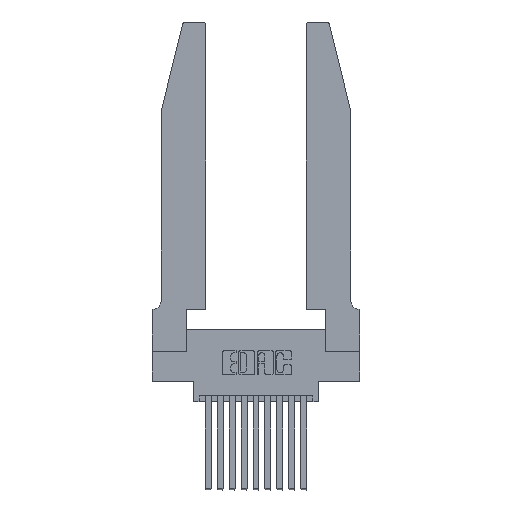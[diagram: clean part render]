
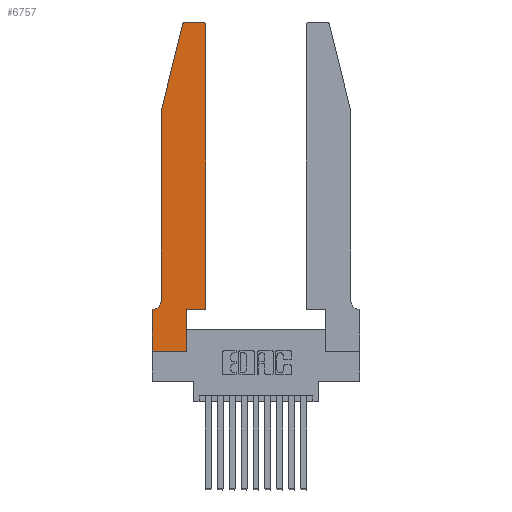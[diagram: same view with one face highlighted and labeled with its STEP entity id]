
A CAD part, top view. The second image highlights one B-rep face of the part: STEP entity #6757.
In plain terms, the highlighted planar face has unit normal (0, 0, 1).
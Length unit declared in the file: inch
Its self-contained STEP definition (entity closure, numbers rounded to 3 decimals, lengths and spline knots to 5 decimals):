
#360 = EDGE_CURVE ( 'NONE', #2141, #6995, #12577, .T. ) ;
#584 = EDGE_CURVE ( 'NONE', #11350, #10825, #13136, .T. ) ;
#772 = VERTEX_POINT ( 'NONE', #2918 ) ;
#892 = VECTOR ( 'NONE', #13113, 39.37008 ) ;
#911 = EDGE_CURVE ( 'NONE', #772, #13180, #12179, .T. ) ;
#1181 = CARTESIAN_POINT ( 'NONE',  ( 0.4205, 2.72, 0.37 ) ) ;
#1663 = DIRECTION ( 'NONE',  ( 0., 1., 0. ) ) ;
#1687 = ORIENTED_EDGE ( 'NONE', *, *, #360, .T. ) ;
#1718 = LINE ( 'NONE', #3929, #2620 ) ;
#1824 = VERTEX_POINT ( 'NONE', #14068 ) ;
#1934 = LINE ( 'NONE', #10554, #11210 ) ;
#2077 = EDGE_CURVE ( 'NONE', #1824, #2141, #7849, .T. ) ;
#2141 = VERTEX_POINT ( 'NONE', #2347 ) ;
#2347 = CARTESIAN_POINT ( 'NONE',  ( 0.4205, 2.75, 0.37 ) ) ;
#2473 = VERTEX_POINT ( 'NONE', #11221 ) ;
#2587 = ORIENTED_EDGE ( 'NONE', *, *, #12162, .T. ) ;
#2606 = CARTESIAN_POINT ( 'NONE',  ( 0.4505, 0.35, 0.37 ) ) ;
#2620 = VECTOR ( 'NONE', #5188, 39.37008 ) ;
#2737 = CARTESIAN_POINT ( 'NONE',  ( 0.0055, 0.42, 0.37 ) ) ;
#2860 = VERTEX_POINT ( 'NONE', #4468 ) ;
#2918 = CARTESIAN_POINT ( 'NONE',  ( 0.0755, 2., 0.37 ) ) ;
#3276 = DIRECTION ( 'NONE',  ( 1., 0., 0. ) ) ;
#3290 = DIRECTION ( 'NONE',  ( 1., 0., 0. ) ) ;
#3381 = CARTESIAN_POINT ( 'NONE',  ( 0.284, 2.72, 0.37 ) ) ;
#3717 = VECTOR ( 'NONE', #14409, 39.37008 ) ;
#3866 = AXIS2_PLACEMENT_3D ( 'NONE', #2737, #11454, #4101 ) ;
#3867 = EDGE_CURVE ( 'NONE', #16018, #772, #12077, .T. ) ;
#3929 = CARTESIAN_POINT ( 'NONE',  ( 0., 0., 0.37 ) ) ;
#4035 = CARTESIAN_POINT ( 'NONE',  ( 0.0755, 2., 0.37 ) ) ;
#4101 = DIRECTION ( 'NONE',  ( -1., 0., 0. ) ) ;
#4468 = CARTESIAN_POINT ( 'NONE',  ( 0.2865, 0.35, 0.37 ) ) ;
#4697 = DIRECTION ( 'NONE',  ( 1., 0., 0. ) ) ;
#4889 = CARTESIAN_POINT ( 'NONE',  ( 0.0755, 0.42, 0.37 ) ) ;
#5188 = DIRECTION ( 'NONE',  ( 0., -1., 0. ) ) ;
#5638 = ORIENTED_EDGE ( 'NONE', *, *, #3867, .T. ) ;
#5704 = VECTOR ( 'NONE', #12519, 39.37008 ) ;
#5881 = EDGE_CURVE ( 'NONE', #2473, #1824, #9596, .T. ) ;
#6305 = VECTOR ( 'NONE', #10790, 39.37008 ) ;
#6439 = ORIENTED_EDGE ( 'NONE', *, *, #584, .T. ) ;
#6757 = ADVANCED_FACE ( 'NONE', ( #13494 ), #14294, .T. ) ;
#6842 = AXIS2_PLACEMENT_3D ( 'NONE', #1181, #14568, #3276 ) ;
#6995 = VERTEX_POINT ( 'NONE', #16111 ) ;
#7089 = LINE ( 'NONE', #13214, #3717 ) ;
#7103 = CARTESIAN_POINT ( 'NONE',  ( 0.0755, 0.35, 0.37 ) ) ;
#7469 = CIRCLE ( 'NONE', #10896, 0.03 ) ;
#7614 = EDGE_CURVE ( 'NONE', #10806, #11350, #1718, .T. ) ;
#7849 = CIRCLE ( 'NONE', #6842, 0.03 ) ;
#8258 = LINE ( 'NONE', #7103, #892 ) ;
#8334 = CARTESIAN_POINT ( 'NONE',  ( 0., 0.35, 0.37 ) ) ;
#8481 = CARTESIAN_POINT ( 'NONE',  ( 0.2605, 2.75, 0.37 ) ) ;
#8576 = ORIENTED_EDGE ( 'NONE', *, *, #13476, .T. ) ;
#8706 = CARTESIAN_POINT ( 'NONE',  ( 0., 0., 0.37 ) ) ;
#8830 = CARTESIAN_POINT ( 'NONE',  ( 0.25487, 2.72718, 0.37 ) ) ;
#8946 = ORIENTED_EDGE ( 'NONE', *, *, #911, .T. ) ;
#9067 = DIRECTION ( 'NONE',  ( -1., 0., 0. ) ) ;
#9222 = VECTOR ( 'NONE', #12546, 39.37008 ) ;
#9330 = ORIENTED_EDGE ( 'NONE', *, *, #12997, .T. ) ;
#9575 = CARTESIAN_POINT ( 'NONE',  ( 0.0755, 2., 0.37 ) ) ;
#9596 = LINE ( 'NONE', #2606, #9222 ) ;
#9603 = CIRCLE ( 'NONE', #3866, 0.07 ) ;
#9933 = CARTESIAN_POINT ( 'NONE',  ( 0., 0.35, 0.37 ) ) ;
#9950 = AXIS2_PLACEMENT_3D ( 'NONE', #8334, #10729, #3290 ) ;
#10070 = ORIENTED_EDGE ( 'NONE', *, *, #13066, .T. ) ;
#10554 = CARTESIAN_POINT ( 'NONE',  ( 0.2865, 0.35, 0.37 ) ) ;
#10729 = DIRECTION ( 'NONE',  ( 0., 0., 1. ) ) ;
#10790 = DIRECTION ( 'NONE',  ( 1., 0., 0. ) ) ;
#10806 = VERTEX_POINT ( 'NONE', #9933 ) ;
#10825 = VERTEX_POINT ( 'NONE', #15928 ) ;
#10896 = AXIS2_PLACEMENT_3D ( 'NONE', #3381, #12016, #4697 ) ;
#10946 = CARTESIAN_POINT ( 'NONE',  ( 0.0055, 0.35, 0.37 ) ) ;
#11210 = VECTOR ( 'NONE', #1663, 39.37008 ) ;
#11221 = CARTESIAN_POINT ( 'NONE',  ( 0.4505, 0.35, 0.37 ) ) ;
#11308 = VERTEX_POINT ( 'NONE', #10946 ) ;
#11350 = VERTEX_POINT ( 'NONE', #8706 ) ;
#11404 = DIRECTION ( 'NONE',  ( -0.239, -0.971, 0. ) ) ;
#11454 = DIRECTION ( 'NONE',  ( 0., 0., -1. ) ) ;
#12016 = DIRECTION ( 'NONE',  ( 0., 0., 1. ) ) ;
#12077 = LINE ( 'NONE', #4035, #15613 ) ;
#12162 = EDGE_CURVE ( 'NONE', #13180, #11308, #9603, .T. ) ;
#12179 = LINE ( 'NONE', #9575, #5704 ) ;
#12505 = ORIENTED_EDGE ( 'NONE', *, *, #7614, .T. ) ;
#12519 = DIRECTION ( 'NONE',  ( 0., -1., 0. ) ) ;
#12546 = DIRECTION ( 'NONE',  ( 0., 1., 0. ) ) ;
#12577 = LINE ( 'NONE', #8481, #15366 ) ;
#12887 = ORIENTED_EDGE ( 'NONE', *, *, #14793, .T. ) ;
#12997 = EDGE_CURVE ( 'NONE', #11308, #10806, #8258, .T. ) ;
#13066 = EDGE_CURVE ( 'NONE', #2860, #2473, #7089, .T. ) ;
#13113 = DIRECTION ( 'NONE',  ( -1., 0., 0. ) ) ;
#13136 = LINE ( 'NONE', #15037, #6305 ) ;
#13180 = VERTEX_POINT ( 'NONE', #4889 ) ;
#13214 = CARTESIAN_POINT ( 'NONE',  ( 0.4505, 0.35, 0.37 ) ) ;
#13256 = ORIENTED_EDGE ( 'NONE', *, *, #5881, .T. ) ;
#13476 = EDGE_CURVE ( 'NONE', #6995, #16018, #7469, .T. ) ;
#13494 = FACE_OUTER_BOUND ( 'NONE', #13653, .T. ) ;
#13635 = ORIENTED_EDGE ( 'NONE', *, *, #2077, .T. ) ;
#13653 = EDGE_LOOP ( 'NONE', ( #1687, #8576, #5638, #8946, #2587, #9330, #12505, #6439, #12887, #10070, #13256, #13635 ) ) ;
#14068 = CARTESIAN_POINT ( 'NONE',  ( 0.4505, 2.72, 0.37 ) ) ;
#14294 = PLANE ( 'NONE',  #9950 ) ;
#14409 = DIRECTION ( 'NONE',  ( 1., 0., 0. ) ) ;
#14568 = DIRECTION ( 'NONE',  ( 0., 0., 1. ) ) ;
#14793 = EDGE_CURVE ( 'NONE', #10825, #2860, #1934, .T. ) ;
#15037 = CARTESIAN_POINT ( 'NONE',  ( 0., 0., 0.37 ) ) ;
#15366 = VECTOR ( 'NONE', #9067, 39.37008 ) ;
#15613 = VECTOR ( 'NONE', #11404, 39.37008 ) ;
#15928 = CARTESIAN_POINT ( 'NONE',  ( 0.2865, 0., 0.37 ) ) ;
#16018 = VERTEX_POINT ( 'NONE', #8830 ) ;
#16111 = CARTESIAN_POINT ( 'NONE',  ( 0.284, 2.75, 0.37 ) ) ;
